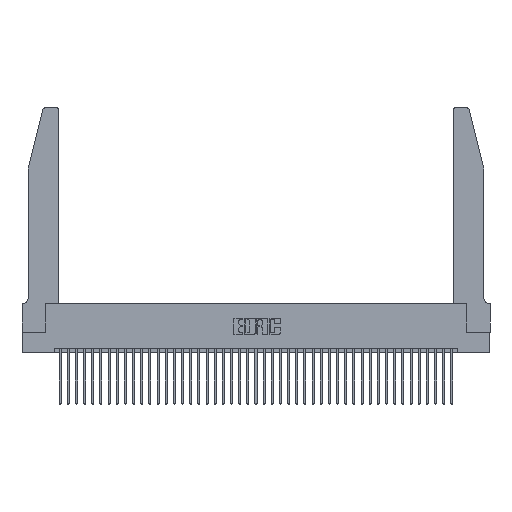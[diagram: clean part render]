
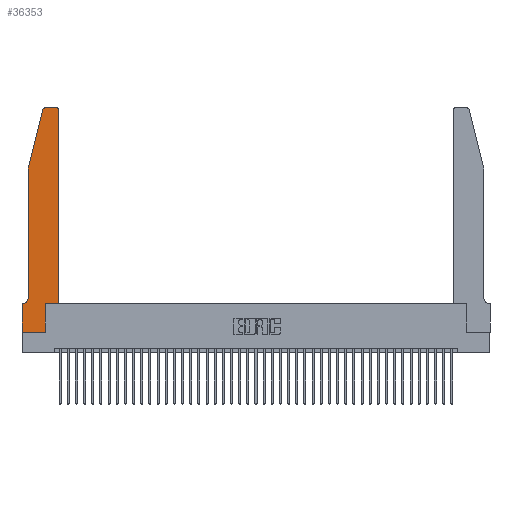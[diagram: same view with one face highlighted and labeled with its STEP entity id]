
A CAD part, top view. The second image highlights one B-rep face of the part: STEP entity #36353.
In plain terms, the highlighted planar face has unit normal (0, 0, 1).
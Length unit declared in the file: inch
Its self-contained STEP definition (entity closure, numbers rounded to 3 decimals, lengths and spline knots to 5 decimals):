
#213 = LINE ( 'NONE', #35077, #16555 ) ;
#541 = EDGE_CURVE ( 'NONE', #40461, #34677, #20726, .T. ) ;
#749 = CARTESIAN_POINT ( 'NONE',  ( 0.0055, 0.42, 0.37 ) ) ;
#1416 = EDGE_CURVE ( 'NONE', #9149, #32685, #213, .T. ) ;
#1962 = VERTEX_POINT ( 'NONE', #26380 ) ;
#2627 = VERTEX_POINT ( 'NONE', #18732 ) ;
#2855 = EDGE_CURVE ( 'NONE', #32685, #15255, #13876, .T. ) ;
#3343 = FACE_OUTER_BOUND ( 'NONE', #16703, .T. ) ;
#3347 = PLANE ( 'NONE',  #39663 ) ;
#3366 = CARTESIAN_POINT ( 'NONE',  ( 0.25487, 2.72718, 0.37 ) ) ;
#3654 = EDGE_CURVE ( 'NONE', #2627, #10284, #13422, .T. ) ;
#3803 = CARTESIAN_POINT ( 'NONE',  ( 0.0755, 2., 0.37 ) ) ;
#3905 = DIRECTION ( 'NONE',  ( -1., 0., 0. ) ) ;
#4316 = ORIENTED_EDGE ( 'NONE', *, *, #41948, .T. ) ;
#5845 = ORIENTED_EDGE ( 'NONE', *, *, #31750, .T. ) ;
#6986 = DIRECTION ( 'NONE',  ( -1., 0., 0. ) ) ;
#7830 = CARTESIAN_POINT ( 'NONE',  ( 0.0755, 0.42, 0.37 ) ) ;
#8254 = ORIENTED_EDGE ( 'NONE', *, *, #20450, .T. ) ;
#8562 = VECTOR ( 'NONE', #6986, 39.37008 ) ;
#9149 = VERTEX_POINT ( 'NONE', #3366 ) ;
#9542 = ORIENTED_EDGE ( 'NONE', *, *, #25676, .T. ) ;
#10284 = VERTEX_POINT ( 'NONE', #12766 ) ;
#11597 = VERTEX_POINT ( 'NONE', #20017 ) ;
#11845 = ORIENTED_EDGE ( 'NONE', *, *, #38611, .T. ) ;
#12636 = ORIENTED_EDGE ( 'NONE', *, *, #29452, .T. ) ;
#12766 = CARTESIAN_POINT ( 'NONE',  ( 0.4505, 2.72, 0.37 ) ) ;
#13422 = LINE ( 'NONE', #23005, #27246 ) ;
#13623 = DIRECTION ( 'NONE',  ( 0., 0., -1. ) ) ;
#13876 = LINE ( 'NONE', #3803, #20026 ) ;
#14590 = EDGE_CURVE ( 'NONE', #15255, #38025, #32806, .T. ) ;
#15255 = VERTEX_POINT ( 'NONE', #7830 ) ;
#16426 = CARTESIAN_POINT ( 'NONE',  ( 0., 0., 0.37 ) ) ;
#16555 = VECTOR ( 'NONE', #25519, 39.37008 ) ;
#16703 = EDGE_LOOP ( 'NONE', ( #4316, #32282, #24809, #37102, #35429, #12636, #34724, #9542, #11845, #8254, #31324, #5845 ) ) ;
#16931 = VECTOR ( 'NONE', #36999, 39.37008 ) ;
#17492 = CARTESIAN_POINT ( 'NONE',  ( 0.0755, 2., 0.37 ) ) ;
#17732 = CARTESIAN_POINT ( 'NONE',  ( 0.4205, 2.75, 0.37 ) ) ;
#17861 = CARTESIAN_POINT ( 'NONE',  ( 0.4205, 2.72, 0.37 ) ) ;
#17972 = CARTESIAN_POINT ( 'NONE',  ( 0., 0., 0.37 ) ) ;
#18251 = CIRCLE ( 'NONE', #32923, 0.03 ) ;
#18732 = CARTESIAN_POINT ( 'NONE',  ( 0.4505, 0.35, 0.37 ) ) ;
#19435 = CARTESIAN_POINT ( 'NONE',  ( 0., 0.35, 0.37 ) ) ;
#20017 = CARTESIAN_POINT ( 'NONE',  ( 0.2865, 0.35, 0.37 ) ) ;
#20026 = VECTOR ( 'NONE', #20069, 39.37008 ) ;
#20069 = DIRECTION ( 'NONE',  ( 0., -1., 0. ) ) ;
#20450 = EDGE_CURVE ( 'NONE', #11597, #2627, #31647, .T. ) ;
#20571 = LINE ( 'NONE', #31148, #28761 ) ;
#20591 = CARTESIAN_POINT ( 'NONE',  ( 0., 0., 0.37 ) ) ;
#20726 = LINE ( 'NONE', #16426, #27921 ) ;
#21029 = DIRECTION ( 'NONE',  ( 0., 1., 0. ) ) ;
#21282 = VECTOR ( 'NONE', #3905, 39.37008 ) ;
#21510 = CARTESIAN_POINT ( 'NONE',  ( 0.0055, 0.35, 0.37 ) ) ;
#21941 = VECTOR ( 'NONE', #30986, 39.37008 ) ;
#22604 = AXIS2_PLACEMENT_3D ( 'NONE', #749, #13623, #36302 ) ;
#23005 = CARTESIAN_POINT ( 'NONE',  ( 0.4505, 0.35, 0.37 ) ) ;
#23640 = CARTESIAN_POINT ( 'NONE',  ( 0.2605, 2.75, 0.37 ) ) ;
#24016 = CARTESIAN_POINT ( 'NONE',  ( 0.2865, 0., 0.37 ) ) ;
#24809 = ORIENTED_EDGE ( 'NONE', *, *, #1416, .T. ) ;
#25519 = DIRECTION ( 'NONE',  ( -0.239, -0.971, 0. ) ) ;
#25676 = EDGE_CURVE ( 'NONE', #34677, #38396, #33295, .T. ) ;
#26380 = CARTESIAN_POINT ( 'NONE',  ( 0.284, 2.75, 0.37 ) ) ;
#27246 = VECTOR ( 'NONE', #39770, 39.37008 ) ;
#27921 = VECTOR ( 'NONE', #35590, 39.37008 ) ;
#27925 = DIRECTION ( 'NONE',  ( 1., 0., 0. ) ) ;
#28761 = VECTOR ( 'NONE', #21029, 39.37008 ) ;
#29144 = AXIS2_PLACEMENT_3D ( 'NONE', #34990, #38560, #38272 ) ;
#29452 = EDGE_CURVE ( 'NONE', #38025, #40461, #32003, .T. ) ;
#29620 = DIRECTION ( 'NONE',  ( 1., 0., 0. ) ) ;
#30706 = CARTESIAN_POINT ( 'NONE',  ( 0.4505, 0.35, 0.37 ) ) ;
#30986 = DIRECTION ( 'NONE',  ( 1., 0., 0. ) ) ;
#31148 = CARTESIAN_POINT ( 'NONE',  ( 0.2865, 0.35, 0.37 ) ) ;
#31324 = ORIENTED_EDGE ( 'NONE', *, *, #3654, .T. ) ;
#31647 = LINE ( 'NONE', #30706, #21941 ) ;
#31750 = EDGE_CURVE ( 'NONE', #10284, #35949, #18251, .T. ) ;
#31898 = CARTESIAN_POINT ( 'NONE',  ( 0., 0.35, 0.37 ) ) ;
#32003 = LINE ( 'NONE', #35999, #21282 ) ;
#32282 = ORIENTED_EDGE ( 'NONE', *, *, #41186, .T. ) ;
#32685 = VERTEX_POINT ( 'NONE', #17492 ) ;
#32806 = CIRCLE ( 'NONE', #22604, 0.07 ) ;
#32923 = AXIS2_PLACEMENT_3D ( 'NONE', #17861, #37897, #27925 ) ;
#33295 = LINE ( 'NONE', #20591, #16931 ) ;
#34677 = VERTEX_POINT ( 'NONE', #17972 ) ;
#34724 = ORIENTED_EDGE ( 'NONE', *, *, #541, .T. ) ;
#34990 = CARTESIAN_POINT ( 'NONE',  ( 0.284, 2.72, 0.37 ) ) ;
#35077 = CARTESIAN_POINT ( 'NONE',  ( 0.0755, 2., 0.37 ) ) ;
#35429 = ORIENTED_EDGE ( 'NONE', *, *, #14590, .T. ) ;
#35590 = DIRECTION ( 'NONE',  ( 0., -1., 0. ) ) ;
#35949 = VERTEX_POINT ( 'NONE', #17732 ) ;
#35999 = CARTESIAN_POINT ( 'NONE',  ( 0.0755, 0.35, 0.37 ) ) ;
#36302 = DIRECTION ( 'NONE',  ( -1., 0., 0. ) ) ;
#36353 = ADVANCED_FACE ( 'NONE', ( #3343 ), #3347, .T. ) ;
#36999 = DIRECTION ( 'NONE',  ( 1., 0., 0. ) ) ;
#37102 = ORIENTED_EDGE ( 'NONE', *, *, #2855, .T. ) ;
#37125 = LINE ( 'NONE', #23640, #8562 ) ;
#37708 = CIRCLE ( 'NONE', #29144, 0.03 ) ;
#37897 = DIRECTION ( 'NONE',  ( 0., 0., 1. ) ) ;
#38025 = VERTEX_POINT ( 'NONE', #21510 ) ;
#38272 = DIRECTION ( 'NONE',  ( 1., 0., 0. ) ) ;
#38396 = VERTEX_POINT ( 'NONE', #24016 ) ;
#38560 = DIRECTION ( 'NONE',  ( 0., 0., 1. ) ) ;
#38611 = EDGE_CURVE ( 'NONE', #38396, #11597, #20571, .T. ) ;
#39663 = AXIS2_PLACEMENT_3D ( 'NONE', #19435, #40979, #29620 ) ;
#39770 = DIRECTION ( 'NONE',  ( 0., 1., 0. ) ) ;
#40461 = VERTEX_POINT ( 'NONE', #31898 ) ;
#40979 = DIRECTION ( 'NONE',  ( 0., 0., 1. ) ) ;
#41186 = EDGE_CURVE ( 'NONE', #1962, #9149, #37708, .T. ) ;
#41948 = EDGE_CURVE ( 'NONE', #35949, #1962, #37125, .T. ) ;
